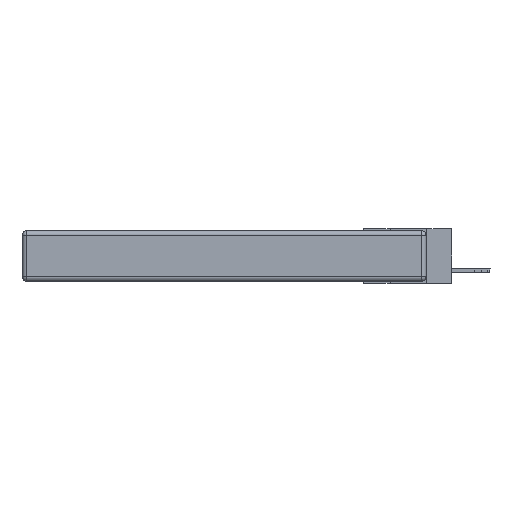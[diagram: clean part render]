
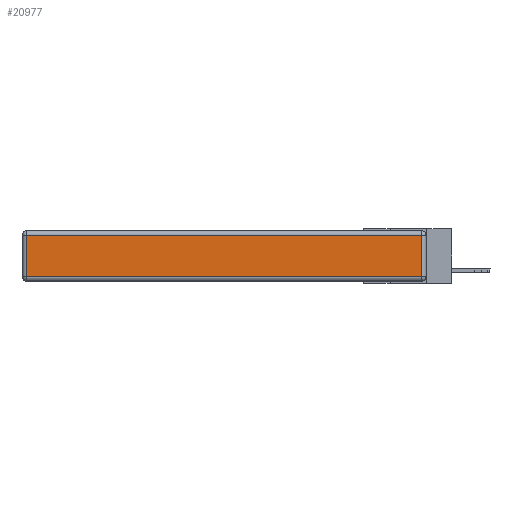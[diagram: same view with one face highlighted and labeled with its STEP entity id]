
A CAD part, left-side view. The second image highlights one B-rep face of the part: STEP entity #20977.
In plain terms, the highlighted planar face has unit normal (-1, 0, 0).
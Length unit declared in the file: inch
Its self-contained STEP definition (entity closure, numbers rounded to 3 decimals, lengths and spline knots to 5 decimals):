
#629 = LINE ( 'NONE', #21386, #21455 ) ;
#917 = DIRECTION ( 'NONE',  ( 0., -1., 0. ) ) ;
#1384 = EDGE_CURVE ( 'NONE', #22077, #20386, #19799, .T. ) ;
#1484 = EDGE_CURVE ( 'NONE', #16517, #15557, #14742, .T. ) ;
#4025 = EDGE_CURVE ( 'NONE', #20386, #16517, #629, .T. ) ;
#4105 = VECTOR ( 'NONE', #9736, 39.37008 ) ;
#5348 = ORIENTED_EDGE ( 'NONE', *, *, #7240, .T. ) ;
#5800 = CARTESIAN_POINT ( 'NONE',  ( 0., 0.03, -0.313 ) ) ;
#5964 = FACE_OUTER_BOUND ( 'NONE', #21101, .T. ) ;
#6808 = DIRECTION ( 'NONE',  ( 0., 0., 1. ) ) ;
#7240 = EDGE_CURVE ( 'NONE', #15557, #22077, #12964, .T. ) ;
#8977 = CARTESIAN_POINT ( 'NONE',  ( 0., 2.72, -0.03 ) ) ;
#9346 = ORIENTED_EDGE ( 'NONE', *, *, #1384, .T. ) ;
#9736 = DIRECTION ( 'NONE',  ( 0., 0., -1. ) ) ;
#9837 = CARTESIAN_POINT ( 'NONE',  ( 0., 2.75, -0.03 ) ) ;
#10282 = VECTOR ( 'NONE', #20836, 39.37008 ) ;
#10348 = CARTESIAN_POINT ( 'NONE',  ( 0., 2.72, -0.313 ) ) ;
#11742 = ORIENTED_EDGE ( 'NONE', *, *, #1484, .T. ) ;
#12414 = ORIENTED_EDGE ( 'NONE', *, *, #4025, .T. ) ;
#12964 = LINE ( 'NONE', #20441, #4105 ) ;
#13334 = CARTESIAN_POINT ( 'NONE',  ( 0., 0., -0.313 ) ) ;
#14742 = LINE ( 'NONE', #9837, #10282 ) ;
#15557 = VERTEX_POINT ( 'NONE', #8977 ) ;
#15629 = PLANE ( 'NONE',  #22459 ) ;
#15851 = DIRECTION ( 'NONE',  ( 0., 0., 1. ) ) ;
#16517 = VERTEX_POINT ( 'NONE', #18653 ) ;
#17031 = CARTESIAN_POINT ( 'NONE',  ( 0., 0., -0.343 ) ) ;
#18646 = VECTOR ( 'NONE', #917, 39.37008 ) ;
#18653 = CARTESIAN_POINT ( 'NONE',  ( 0., 0.03, -0.03 ) ) ;
#19799 = LINE ( 'NONE', #13334, #18646 ) ;
#20386 = VERTEX_POINT ( 'NONE', #5800 ) ;
#20441 = CARTESIAN_POINT ( 'NONE',  ( 0., 2.72, -0.343 ) ) ;
#20836 = DIRECTION ( 'NONE',  ( 0., 1., 0. ) ) ;
#20977 = ADVANCED_FACE ( 'NONE', ( #5964 ), #15629, .T. ) ;
#21101 = EDGE_LOOP ( 'NONE', ( #9346, #12414, #11742, #5348 ) ) ;
#21169 = DIRECTION ( 'NONE',  ( -1., 0., 0. ) ) ;
#21386 = CARTESIAN_POINT ( 'NONE',  ( 0., 0.03, -0.343 ) ) ;
#21455 = VECTOR ( 'NONE', #15851, 39.37008 ) ;
#22077 = VERTEX_POINT ( 'NONE', #10348 ) ;
#22459 = AXIS2_PLACEMENT_3D ( 'NONE', #17031, #21169, #6808 ) ;
